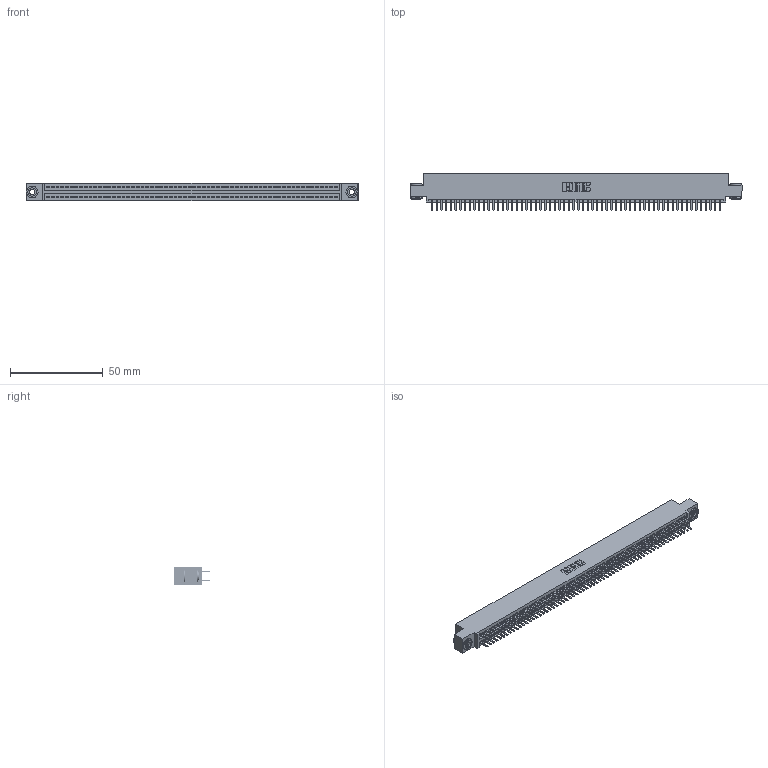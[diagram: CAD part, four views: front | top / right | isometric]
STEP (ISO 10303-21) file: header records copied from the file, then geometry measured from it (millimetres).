
FILE_DESCRIPTION (( 'STEP AP203' ), '1' );
FILE_NAME ('845-124-520-503.STEP', '2018-11-21T16:39:43', ( '' ), ( '' ), 'SwSTEP 2.0', 'SolidWorks 2016', '' );
FILE_SCHEMA (( 'CONFIG_CONTROL_DESIGN' ));
Length unit declared in the file: inch
Products named in the file (4): 845 Part_0.110 Offset - 0.156 Dia-TH; 345-292-001_345-293-120; 345-250-002_345-250-002-102; 845-124-520-503
Assembly tree (127 placements, depth 2):
  845-124-520-503
    845 Part_0.110 Offset - 0.156 Dia-TH
    345-292-001_345-293-120  x124
    345-250-002_345-250-002-102  x2
Bounding box: 178.69 x 19.68 x 9.4 mm (x, y, z)
Volume: 17435.2 mm3; surface area: 26341.3 mm2
Topology: 127 solids, 127 shells, 6864 faces, 19897 edges, 12930 vertices
Faces by surface type: plane 4434, cylinder 2422, cone 8
Entity records: 46850 total; most frequent: CARTESIAN_POINT 7823, ORIENTED_EDGE 7738, DIRECTION 6891, EDGE_CURVE 3869, LINE 3461, VECTOR 3461, VERTEX_POINT 2574, AXIS2_PLACEMENT_3D 1715
